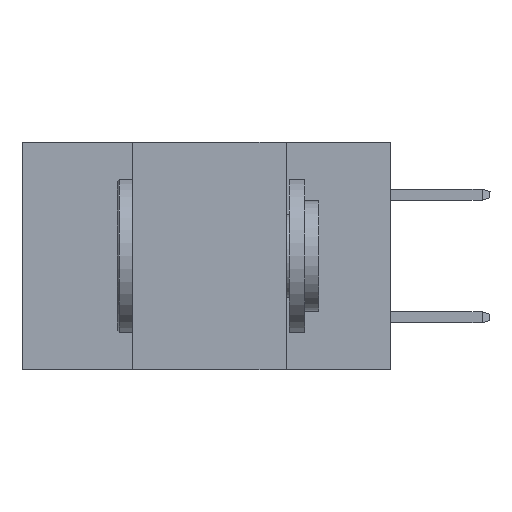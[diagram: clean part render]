
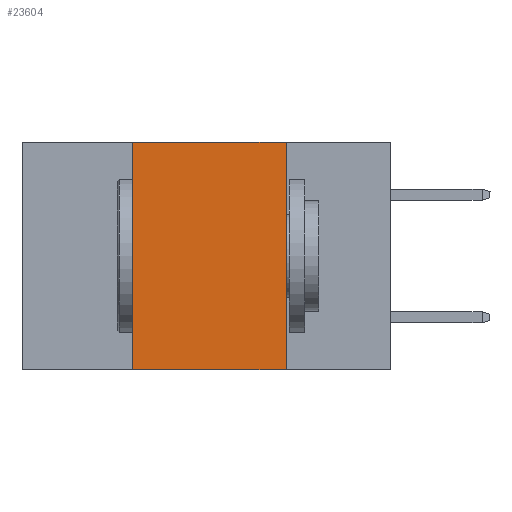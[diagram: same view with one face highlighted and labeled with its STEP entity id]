
A CAD part, left-side view. The second image highlights one B-rep face of the part: STEP entity #23604.
In plain terms, the highlighted planar face has unit normal (-1, 0, 0).
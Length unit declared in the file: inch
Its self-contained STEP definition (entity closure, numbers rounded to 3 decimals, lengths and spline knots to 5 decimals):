
#2060 = CARTESIAN_POINT ( 'NONE',  ( 0., 0.17, 0. ) ) ;
#2303 = AXIS2_PLACEMENT_3D ( 'NONE', #27880, #10893, #37911 ) ;
#2687 = EDGE_CURVE ( 'NONE', #36132, #15016, #8502, .T. ) ;
#4290 = VECTOR ( 'NONE', #30261, 39.37008 ) ;
#6036 = ORIENTED_EDGE ( 'NONE', *, *, #12009, .T. ) ;
#6802 = LINE ( 'NONE', #6856, #19384 ) ;
#6856 = CARTESIAN_POINT ( 'NONE',  ( 0., 0.6, 0. ) ) ;
#7214 = ORIENTED_EDGE ( 'NONE', *, *, #2687, .F. ) ;
#8502 = LINE ( 'NONE', #16721, #4290 ) ;
#9494 = DIRECTION ( 'NONE',  ( 0., 0., -1. ) ) ;
#10226 = EDGE_CURVE ( 'NONE', #15016, #27249, #6802, .T. ) ;
#10893 = DIRECTION ( 'NONE',  ( 1., 0., 0. ) ) ;
#12009 = EDGE_CURVE ( 'NONE', #36132, #29449, #26213, .T. ) ;
#12107 = ORIENTED_EDGE ( 'NONE', *, *, #10226, .F. ) ;
#13429 = FACE_OUTER_BOUND ( 'NONE', #32937, .T. ) ;
#14891 = PLANE ( 'NONE',  #2303 ) ;
#15016 = VERTEX_POINT ( 'NONE', #16128 ) ;
#16126 = CARTESIAN_POINT ( 'NONE',  ( 0., 0.17, 0. ) ) ;
#16128 = CARTESIAN_POINT ( 'NONE',  ( 0., 0.42, 0. ) ) ;
#16721 = CARTESIAN_POINT ( 'NONE',  ( 0., 0.42, 0. ) ) ;
#18737 = VECTOR ( 'NONE', #9494, 39.37008 ) ;
#19384 = VECTOR ( 'NONE', #23499, 39.37008 ) ;
#20298 = LINE ( 'NONE', #2060, #18737 ) ;
#23035 = EDGE_CURVE ( 'NONE', #27249, #29449, #20298, .T. ) ;
#23499 = DIRECTION ( 'NONE',  ( 0., -1., 0. ) ) ;
#23604 = ADVANCED_FACE ( 'NONE', ( #13429 ), #14891, .F. ) ;
#24355 = CARTESIAN_POINT ( 'NONE',  ( 0., 0.42, -0.37 ) ) ;
#26213 = LINE ( 'NONE', #43252, #42012 ) ;
#27249 = VERTEX_POINT ( 'NONE', #16126 ) ;
#27880 = CARTESIAN_POINT ( 'NONE',  ( 0., 0.6, 0. ) ) ;
#29449 = VERTEX_POINT ( 'NONE', #35146 ) ;
#30261 = DIRECTION ( 'NONE',  ( 0., 0., 1. ) ) ;
#32937 = EDGE_LOOP ( 'NONE', ( #36595, #12107, #7214, #6036 ) ) ;
#33307 = DIRECTION ( 'NONE',  ( 0., -1., 0. ) ) ;
#35146 = CARTESIAN_POINT ( 'NONE',  ( 0., 0.17, -0.37 ) ) ;
#36132 = VERTEX_POINT ( 'NONE', #24355 ) ;
#36595 = ORIENTED_EDGE ( 'NONE', *, *, #23035, .F. ) ;
#37911 = DIRECTION ( 'NONE',  ( 0., 0., -1. ) ) ;
#42012 = VECTOR ( 'NONE', #33307, 39.37008 ) ;
#43252 = CARTESIAN_POINT ( 'NONE',  ( 0., 0.6, -0.37 ) ) ;
